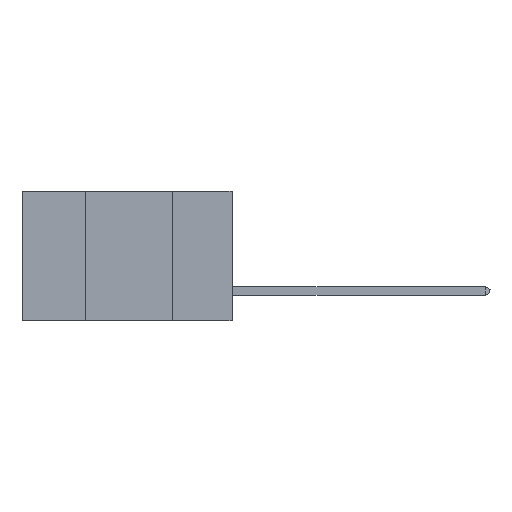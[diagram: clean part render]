
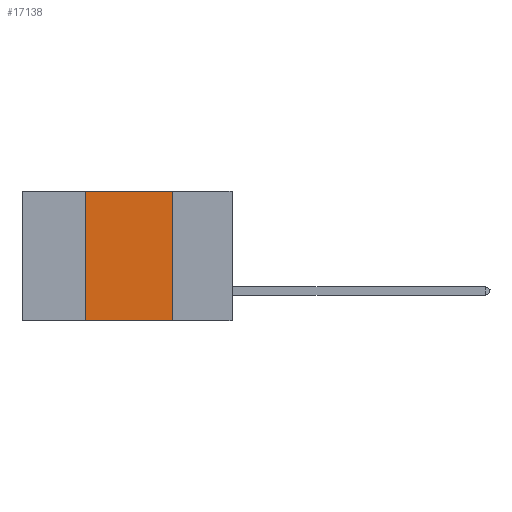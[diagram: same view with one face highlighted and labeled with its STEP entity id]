
A CAD part, left-side view. The second image highlights one B-rep face of the part: STEP entity #17138.
In plain terms, the highlighted planar face has unit normal (-1, 0, 0).
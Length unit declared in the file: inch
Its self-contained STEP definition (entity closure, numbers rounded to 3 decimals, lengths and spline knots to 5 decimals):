
#512 = VERTEX_POINT ( 'NONE', #11539 ) ;
#576 = EDGE_CURVE ( 'NONE', #14992, #3041, #5334, .T. ) ;
#1133 = CARTESIAN_POINT ( 'NONE',  ( 0., 0.6, 0. ) ) ;
#1272 = DIRECTION ( 'NONE',  ( 0., 0., -1. ) ) ;
#1546 = CARTESIAN_POINT ( 'NONE',  ( 0., 0.17, -0.37 ) ) ;
#2153 = ORIENTED_EDGE ( 'NONE', *, *, #11913, .F. ) ;
#2298 = DIRECTION ( 'NONE',  ( 1., 0., 0. ) ) ;
#2612 = ORIENTED_EDGE ( 'NONE', *, *, #7271, .T. ) ;
#2613 = ORIENTED_EDGE ( 'NONE', *, *, #576, .F. ) ;
#2949 = EDGE_LOOP ( 'NONE', ( #2613, #2153, #5916, #2612 ) ) ;
#3041 = VERTEX_POINT ( 'NONE', #1546 ) ;
#3352 = CARTESIAN_POINT ( 'NONE',  ( 0., 0.6, -0.37 ) ) ;
#4682 = DIRECTION ( 'NONE',  ( 0., -1., 0. ) ) ;
#4917 = VECTOR ( 'NONE', #1272, 39.37008 ) ;
#5262 = DIRECTION ( 'NONE',  ( 0., -1., 0. ) ) ;
#5334 = LINE ( 'NONE', #9247, #4917 ) ;
#5916 = ORIENTED_EDGE ( 'NONE', *, *, #15237, .F. ) ;
#6700 = CARTESIAN_POINT ( 'NONE',  ( 0., 0.42, 0. ) ) ;
#6878 = VECTOR ( 'NONE', #4682, 39.37008 ) ;
#7271 = EDGE_CURVE ( 'NONE', #512, #3041, #11125, .T. ) ;
#7538 = CARTESIAN_POINT ( 'NONE',  ( 0., 0.6, 0. ) ) ;
#9247 = CARTESIAN_POINT ( 'NONE',  ( 0., 0.17, 0. ) ) ;
#9330 = VECTOR ( 'NONE', #10670, 39.37008 ) ;
#10196 = DIRECTION ( 'NONE',  ( 0., 0., -1. ) ) ;
#10259 = CARTESIAN_POINT ( 'NONE',  ( 0., 0.17, 0. ) ) ;
#10411 = AXIS2_PLACEMENT_3D ( 'NONE', #7538, #2298, #10196 ) ;
#10670 = DIRECTION ( 'NONE',  ( 0., 0., 1. ) ) ;
#10829 = CARTESIAN_POINT ( 'NONE',  ( 0., 0.42, 0. ) ) ;
#11125 = LINE ( 'NONE', #3352, #6878 ) ;
#11539 = CARTESIAN_POINT ( 'NONE',  ( 0., 0.42, -0.37 ) ) ;
#11799 = PLANE ( 'NONE',  #10411 ) ;
#11913 = EDGE_CURVE ( 'NONE', #12691, #14992, #12405, .T. ) ;
#12405 = LINE ( 'NONE', #1133, #16837 ) ;
#12691 = VERTEX_POINT ( 'NONE', #10829 ) ;
#14992 = VERTEX_POINT ( 'NONE', #10259 ) ;
#15215 = FACE_OUTER_BOUND ( 'NONE', #2949, .T. ) ;
#15237 = EDGE_CURVE ( 'NONE', #512, #12691, #15911, .T. ) ;
#15911 = LINE ( 'NONE', #6700, #9330 ) ;
#16837 = VECTOR ( 'NONE', #5262, 39.37008 ) ;
#17138 = ADVANCED_FACE ( 'NONE', ( #15215 ), #11799, .F. ) ;
